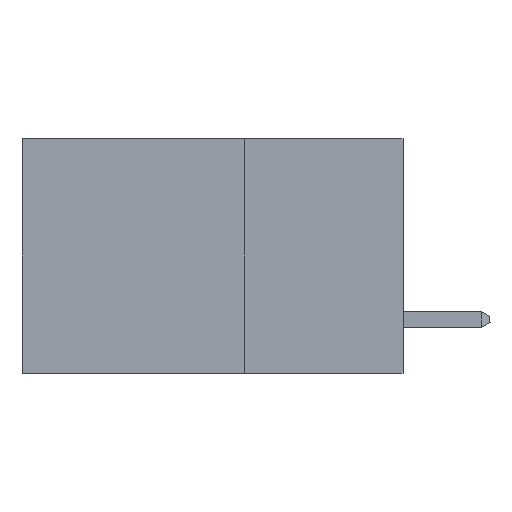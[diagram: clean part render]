
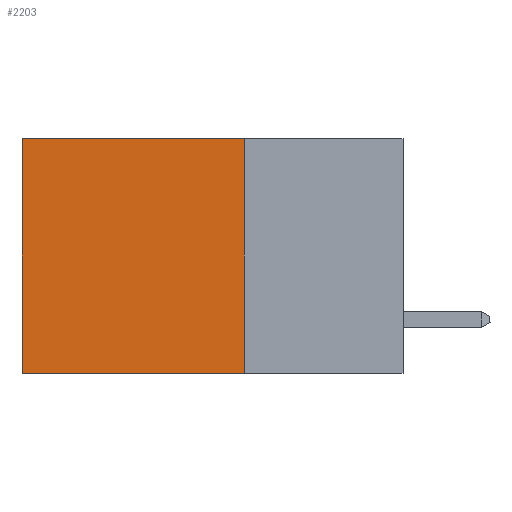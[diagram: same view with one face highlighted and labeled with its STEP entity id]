
A CAD part, left-side view. The second image highlights one B-rep face of the part: STEP entity #2203.
In plain terms, the highlighted planar face has unit normal (-1, 0, 0).
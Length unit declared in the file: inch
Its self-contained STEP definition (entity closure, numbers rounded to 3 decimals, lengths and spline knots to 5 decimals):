
#715 = ORIENTED_EDGE ( 'NONE', *, *, #5227, .F. ) ;
#912 = ORIENTED_EDGE ( 'NONE', *, *, #2387, .F. ) ;
#1277 = ORIENTED_EDGE ( 'NONE', *, *, #10893, .T. ) ;
#1527 = CARTESIAN_POINT ( 'NONE',  ( 0.2875, 0.25, 0. ) ) ;
#1637 = EDGE_CURVE ( 'NONE', #11286, #9518, #1719, .T. ) ;
#1719 = LINE ( 'NONE', #1998, #13644 ) ;
#1998 = CARTESIAN_POINT ( 'NONE',  ( 0.2875, 0.6, 0. ) ) ;
#2203 = ADVANCED_FACE ( 'NONE', ( #11463 ), #2483, .F. ) ;
#2387 = EDGE_CURVE ( 'NONE', #8473, #14620, #12716, .T. ) ;
#2483 = PLANE ( 'NONE',  #3611 ) ;
#3396 = DIRECTION ( 'NONE',  ( 0., 1., 0. ) ) ;
#3611 = AXIS2_PLACEMENT_3D ( 'NONE', #8191, #4935, #9312 ) ;
#3890 = CARTESIAN_POINT ( 'NONE',  ( 0.2875, 0.25, -0.37 ) ) ;
#4935 = DIRECTION ( 'NONE',  ( 1., 0., 0. ) ) ;
#5227 = EDGE_CURVE ( 'NONE', #14620, #9518, #14458, .T. ) ;
#7049 = CARTESIAN_POINT ( 'NONE',  ( 0.2875, 0.25, 0. ) ) ;
#7797 = LINE ( 'NONE', #7049, #9394 ) ;
#8191 = CARTESIAN_POINT ( 'NONE',  ( 0.2875, 0.25, 0. ) ) ;
#8339 = CARTESIAN_POINT ( 'NONE',  ( 0.2875, 0.6, -0.37 ) ) ;
#8473 = VERTEX_POINT ( 'NONE', #9787 ) ;
#9312 = DIRECTION ( 'NONE',  ( 0., 0., -1. ) ) ;
#9394 = VECTOR ( 'NONE', #3396, 39.37008 ) ;
#9518 = VERTEX_POINT ( 'NONE', #8339 ) ;
#9567 = DIRECTION ( 'NONE',  ( 0., 0., -1. ) ) ;
#9726 = VECTOR ( 'NONE', #10737, 39.37008 ) ;
#9787 = CARTESIAN_POINT ( 'NONE',  ( 0.2875, 0.25, 0. ) ) ;
#10052 = DIRECTION ( 'NONE',  ( 0., 0., -1. ) ) ;
#10360 = VECTOR ( 'NONE', #9567, 39.37008 ) ;
#10737 = DIRECTION ( 'NONE',  ( 0., 1., 0. ) ) ;
#10893 = EDGE_CURVE ( 'NONE', #8473, #11286, #7797, .T. ) ;
#11272 = CARTESIAN_POINT ( 'NONE',  ( 0.2875, 0.6, 0. ) ) ;
#11286 = VERTEX_POINT ( 'NONE', #11272 ) ;
#11463 = FACE_OUTER_BOUND ( 'NONE', #14435, .T. ) ;
#11706 = CARTESIAN_POINT ( 'NONE',  ( 0.2875, 0.25, -0.37 ) ) ;
#12716 = LINE ( 'NONE', #1527, #10360 ) ;
#12730 = ORIENTED_EDGE ( 'NONE', *, *, #1637, .T. ) ;
#13644 = VECTOR ( 'NONE', #10052, 39.37008 ) ;
#14435 = EDGE_LOOP ( 'NONE', ( #12730, #715, #912, #1277 ) ) ;
#14458 = LINE ( 'NONE', #3890, #9726 ) ;
#14620 = VERTEX_POINT ( 'NONE', #11706 ) ;
